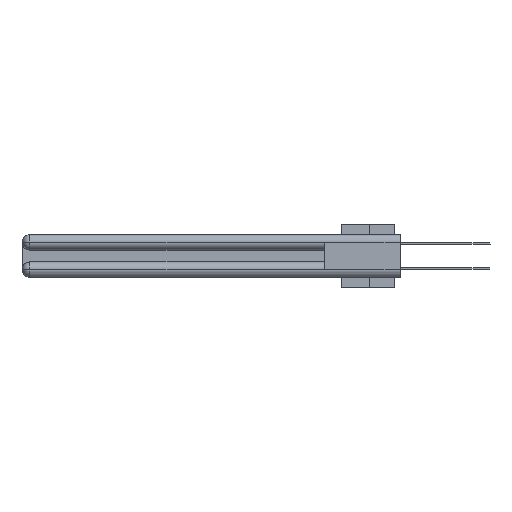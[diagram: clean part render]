
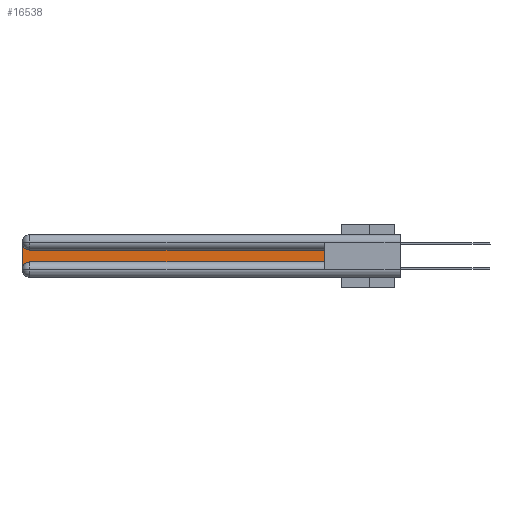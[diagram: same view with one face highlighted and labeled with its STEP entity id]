
A CAD part, left-side view. The second image highlights one B-rep face of the part: STEP entity #16538.
In plain terms, the highlighted planar face has unit normal (-1, 0, 0).
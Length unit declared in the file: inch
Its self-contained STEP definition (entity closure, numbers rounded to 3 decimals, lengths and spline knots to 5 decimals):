
#1766 = DIRECTION ( 'NONE',  ( 1., 0., 0. ) ) ;
#2502 = DIRECTION ( 'NONE',  ( 1., 0., 0. ) ) ;
#3108 = DIRECTION ( 'NONE',  ( 0., 1., 0. ) ) ;
#3642 = EDGE_CURVE ( 'NONE', #18838, #7633, #19234, .T. ) ;
#5065 = EDGE_CURVE ( 'NONE', #18906, #14355, #11341, .T. ) ;
#6765 = CARTESIAN_POINT ( 'NONE',  ( 0.075, 3., -0.2175 ) ) ;
#7633 = VERTEX_POINT ( 'NONE', #32049 ) ;
#8037 = DIRECTION ( 'NONE',  ( 0., -1., 0. ) ) ;
#8388 = DIRECTION ( 'NONE',  ( 0., 0., -1. ) ) ;
#8459 = LINE ( 'NONE', #10022, #17607 ) ;
#8570 = VERTEX_POINT ( 'NONE', #8818 ) ;
#8818 = CARTESIAN_POINT ( 'NONE',  ( 0.075, 3., -0.2775 ) ) ;
#10022 = CARTESIAN_POINT ( 'NONE',  ( 0.075, 0.6, -0.2175 ) ) ;
#10353 = CARTESIAN_POINT ( 'NONE',  ( 0.075, 3., -0.1225 ) ) ;
#10915 = CARTESIAN_POINT ( 'NONE',  ( 0.075, 2.94, -0.2175 ) ) ;
#11341 = LINE ( 'NONE', #11491, #12232 ) ;
#11491 = CARTESIAN_POINT ( 'NONE',  ( 0.075, 0.6, -0.1225 ) ) ;
#12232 = VECTOR ( 'NONE', #3108, 39.37008 ) ;
#12490 = CARTESIAN_POINT ( 'NONE',  ( 0.075, 2.94, -0.1225 ) ) ;
#13749 = ORIENTED_EDGE ( 'NONE', *, *, #16369, .T. ) ;
#14355 = VERTEX_POINT ( 'NONE', #12490 ) ;
#16369 = EDGE_CURVE ( 'NONE', #22812, #8570, #22282, .T. ) ;
#16538 = ADVANCED_FACE ( 'NONE', ( #27761 ), #36370, .F. ) ;
#17284 = CARTESIAN_POINT ( 'NONE',  ( 0.075, 2.94, -0.0625 ) ) ;
#17607 = VECTOR ( 'NONE', #30723, 39.37008 ) ;
#18494 = ORIENTED_EDGE ( 'NONE', *, *, #34264, .T. ) ;
#18838 = VERTEX_POINT ( 'NONE', #10915 ) ;
#18906 = VERTEX_POINT ( 'NONE', #25087 ) ;
#19209 = AXIS2_PLACEMENT_3D ( 'NONE', #10353, #1766, #36630 ) ;
#19234 = LINE ( 'NONE', #28167, #21050 ) ;
#19697 = EDGE_CURVE ( 'NONE', #7633, #18906, #8459, .T. ) ;
#20337 = EDGE_CURVE ( 'NONE', #8570, #18838, #32600, .T. ) ;
#21050 = VECTOR ( 'NONE', #8037, 39.37008 ) ;
#22282 = LINE ( 'NONE', #6765, #31842 ) ;
#22812 = VERTEX_POINT ( 'NONE', #23710 ) ;
#23710 = CARTESIAN_POINT ( 'NONE',  ( 0.075, 3., -0.0625 ) ) ;
#24386 = EDGE_LOOP ( 'NONE', ( #37211, #18494, #13749, #31993, #37361, #37259 ) ) ;
#25087 = CARTESIAN_POINT ( 'NONE',  ( 0.075, 0.6, -0.1225 ) ) ;
#26103 = CARTESIAN_POINT ( 'NONE',  ( 0.075, 2.94, -0.2775 ) ) ;
#26859 = CIRCLE ( 'NONE', #30396, 0.06 ) ;
#27761 = FACE_OUTER_BOUND ( 'NONE', #24386, .T. ) ;
#28167 = CARTESIAN_POINT ( 'NONE',  ( 0.075, 0.6, -0.2175 ) ) ;
#28994 = DIRECTION ( 'NONE',  ( 1., 0., 0. ) ) ;
#30396 = AXIS2_PLACEMENT_3D ( 'NONE', #17284, #28994, #37643 ) ;
#30723 = DIRECTION ( 'NONE',  ( 0., 0., 1. ) ) ;
#31526 = AXIS2_PLACEMENT_3D ( 'NONE', #26103, #2502, #8388 ) ;
#31842 = VECTOR ( 'NONE', #35732, 39.37008 ) ;
#31993 = ORIENTED_EDGE ( 'NONE', *, *, #20337, .T. ) ;
#32049 = CARTESIAN_POINT ( 'NONE',  ( 0.075, 0.6, -0.2175 ) ) ;
#32600 = CIRCLE ( 'NONE', #31526, 0.06 ) ;
#34264 = EDGE_CURVE ( 'NONE', #14355, #22812, #26859, .T. ) ;
#35732 = DIRECTION ( 'NONE',  ( 0., 0., -1. ) ) ;
#36370 = PLANE ( 'NONE',  #19209 ) ;
#36630 = DIRECTION ( 'NONE',  ( 0., 0., -1. ) ) ;
#37211 = ORIENTED_EDGE ( 'NONE', *, *, #5065, .T. ) ;
#37259 = ORIENTED_EDGE ( 'NONE', *, *, #19697, .T. ) ;
#37361 = ORIENTED_EDGE ( 'NONE', *, *, #3642, .T. ) ;
#37643 = DIRECTION ( 'NONE',  ( 0., 0., -1. ) ) ;
